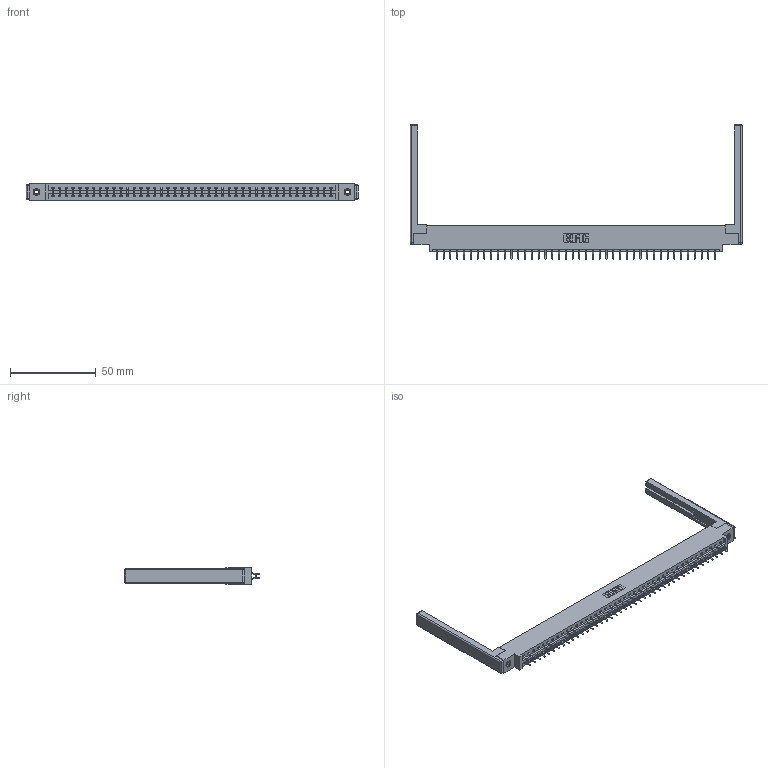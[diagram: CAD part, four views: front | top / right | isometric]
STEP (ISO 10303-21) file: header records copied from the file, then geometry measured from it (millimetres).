
FILE_DESCRIPTION (( 'STEP AP203' ), '1' );
FILE_NAME ('387-084-556-868.STEP', '2019-10-23T02:12:09', ( '' ), ( '' ), 'SwSTEP 2.0', 'SolidWorks 2016', '' );
FILE_SCHEMA (( 'CONFIG_CONTROL_DESIGN' ));
Length unit declared in the file: inch
Products named in the file (5): 307-220-068; 337 Part_0.170 Offset - 0.156 Dia-TI; 345-250-001_345-250-001-102; 345-292-001_556 Tail; 387-084-556-868
Assembly tree (89 placements, depth 2):
  387-084-556-868
    337 Part_0.170 Offset - 0.156 Dia-TI
    345-292-001_556 Tail  x84
    345-250-001_345-250-001-102  x2
    307-220-068  x2
Bounding box: 193.85 x 78.63 x 9.4 mm (x, y, z)
Volume: 24693.7 mm3; surface area: 27012.8 mm2
Topology: 89 solids, 89 shells, 5312 faces, 15749 edges, 10366 vertices
Faces by surface type: plane 3690, cylinder 1598, cone 12, sphere 8, torus 4
Entity records: 35676 total; most frequent: CARTESIAN_POINT 5991, ORIENTED_EDGE 5904, DIRECTION 5154, EDGE_CURVE 2952, VECTOR 2766, LINE 2766, VERTEX_POINT 1958, AXIS2_PLACEMENT_3D 1194
